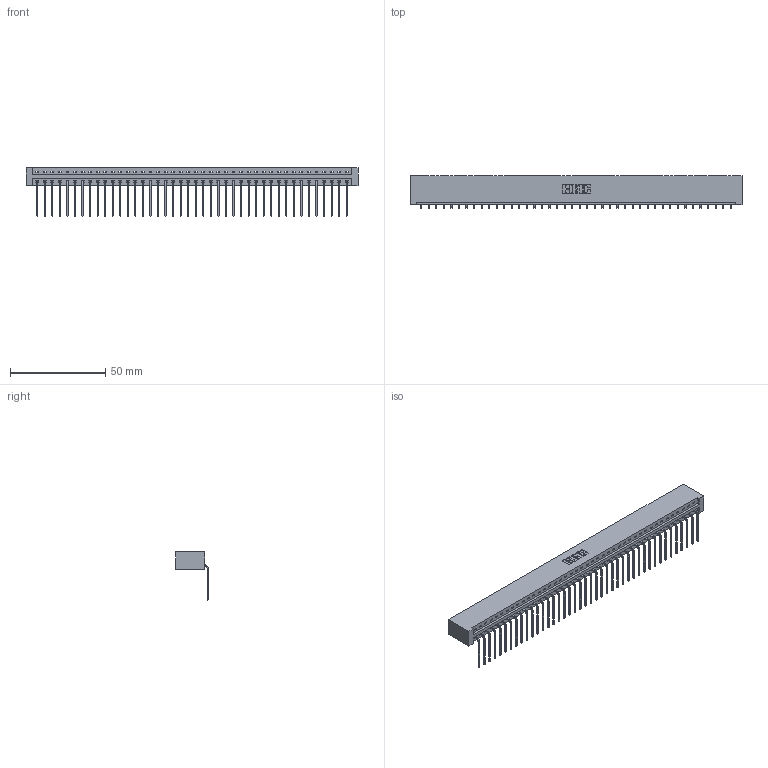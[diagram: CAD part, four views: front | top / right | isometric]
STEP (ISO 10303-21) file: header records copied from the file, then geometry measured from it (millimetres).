
FILE_DESCRIPTION (( 'STEP AP203' ), '1' );
FILE_NAME ('337-042-559-101.STEP', '2018-08-09T01:51:16', ( '' ), ( '' ), 'SwSTEP 2.0', 'SolidWorks 2016', '' );
FILE_SCHEMA (( 'CONFIG_CONTROL_DESIGN' ));
Length unit declared in the file: inch
Products named in the file (3): 337 Part_No Mounting Lugs; 345-292-001_558 559 Tail - 1; 337-042-559-101
Assembly tree (43 placements, depth 2):
  337-042-559-101
    337 Part_No Mounting Lugs
    345-292-001_558 559 Tail - 1  x42
Bounding box: 174.29 x 17.09 x 25.53 mm (x, y, z)
Volume: 18993.7 mm3; surface area: 20468.3 mm2
Topology: 43 solids, 43 shells, 2794 faces, 8435 edges, 5566 vertices
Faces by surface type: plane 2082, cylinder 712
Entity records: 31027 total; most frequent: CARTESIAN_POINT 5412, ORIENTED_EDGE 5390, DIRECTION 4547, EDGE_CURVE 2695, VECTOR 2575, LINE 2575, VERTEX_POINT 1794, AXIS2_PLACEMENT_3D 986
